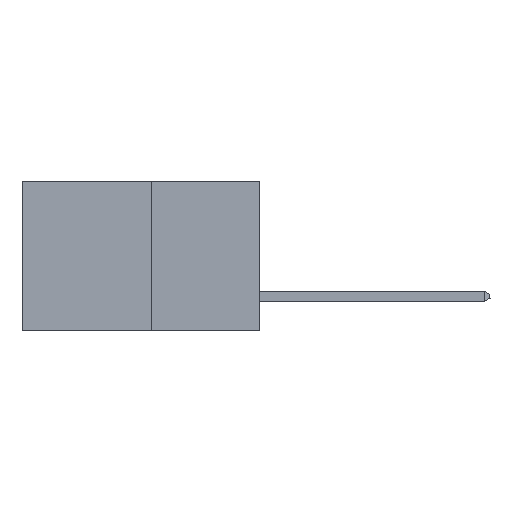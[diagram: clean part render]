
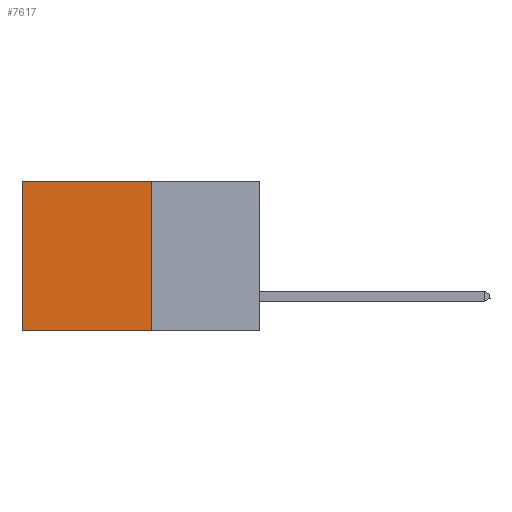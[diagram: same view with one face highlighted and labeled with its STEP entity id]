
A CAD part, left-side view. The second image highlights one B-rep face of the part: STEP entity #7617.
In plain terms, the highlighted planar face has unit normal (-1, 0, 0).
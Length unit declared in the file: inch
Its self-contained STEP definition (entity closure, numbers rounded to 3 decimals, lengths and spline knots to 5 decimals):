
#698 = CARTESIAN_POINT ( 'NONE',  ( 0.277, 0.27, -0.37 ) ) ;
#899 = VERTEX_POINT ( 'NONE', #14447 ) ;
#1241 = ORIENTED_EDGE ( 'NONE', *, *, #6517, .T. ) ;
#1296 = LINE ( 'NONE', #13320, #7712 ) ;
#1622 = ORIENTED_EDGE ( 'NONE', *, *, #2816, .F. ) ;
#1681 = LINE ( 'NONE', #3751, #14515 ) ;
#2014 = PLANE ( 'NONE',  #12595 ) ;
#2324 = VECTOR ( 'NONE', #11799, 39.37008 ) ;
#2750 = VERTEX_POINT ( 'NONE', #5851 ) ;
#2816 = EDGE_CURVE ( 'NONE', #6248, #2750, #1296, .T. ) ;
#3228 = CARTESIAN_POINT ( 'NONE',  ( 0.277, 0.27, -0.37 ) ) ;
#3294 = DIRECTION ( 'NONE',  ( 0., 0., -1. ) ) ;
#3751 = CARTESIAN_POINT ( 'NONE',  ( 0.277, 0.59, -0.37 ) ) ;
#5056 = CARTESIAN_POINT ( 'NONE',  ( 0.277, 0.27, 0. ) ) ;
#5851 = CARTESIAN_POINT ( 'NONE',  ( 0.277, 0.59, -0.37 ) ) ;
#6248 = VERTEX_POINT ( 'NONE', #3228 ) ;
#6324 = DIRECTION ( 'NONE',  ( 0., 1., 0. ) ) ;
#6517 = EDGE_CURVE ( 'NONE', #15669, #899, #12933, .T. ) ;
#7246 = DIRECTION ( 'NONE',  ( 0., 1., 0. ) ) ;
#7617 = ADVANCED_FACE ( 'NONE', ( #9864 ), #2014, .F. ) ;
#7712 = VECTOR ( 'NONE', #7246, 39.37008 ) ;
#8985 = EDGE_CURVE ( 'NONE', #15669, #6248, #12328, .T. ) ;
#9864 = FACE_OUTER_BOUND ( 'NONE', #16143, .T. ) ;
#10804 = DIRECTION ( 'NONE',  ( 1., 0., 0. ) ) ;
#11799 = DIRECTION ( 'NONE',  ( 0., 0., -1. ) ) ;
#12328 = LINE ( 'NONE', #13019, #2324 ) ;
#12344 = CARTESIAN_POINT ( 'NONE',  ( 0.277, 0.27, 0. ) ) ;
#12595 = AXIS2_PLACEMENT_3D ( 'NONE', #698, #10804, #3294 ) ;
#12933 = LINE ( 'NONE', #5056, #16107 ) ;
#13019 = CARTESIAN_POINT ( 'NONE',  ( 0.277, 0.27, -0.37 ) ) ;
#13320 = CARTESIAN_POINT ( 'NONE',  ( 0.277, 0.27, -0.37 ) ) ;
#14447 = CARTESIAN_POINT ( 'NONE',  ( 0.277, 0.59, 0. ) ) ;
#14515 = VECTOR ( 'NONE', #14874, 39.37008 ) ;
#14874 = DIRECTION ( 'NONE',  ( 0., 0., -1. ) ) ;
#15043 = ORIENTED_EDGE ( 'NONE', *, *, #8985, .F. ) ;
#15669 = VERTEX_POINT ( 'NONE', #12344 ) ;
#15975 = EDGE_CURVE ( 'NONE', #899, #2750, #1681, .T. ) ;
#16018 = ORIENTED_EDGE ( 'NONE', *, *, #15975, .T. ) ;
#16107 = VECTOR ( 'NONE', #6324, 39.37008 ) ;
#16143 = EDGE_LOOP ( 'NONE', ( #16018, #1622, #15043, #1241 ) ) ;
